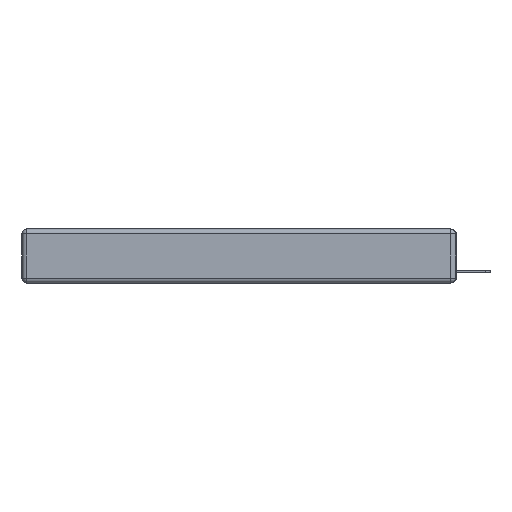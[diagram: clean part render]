
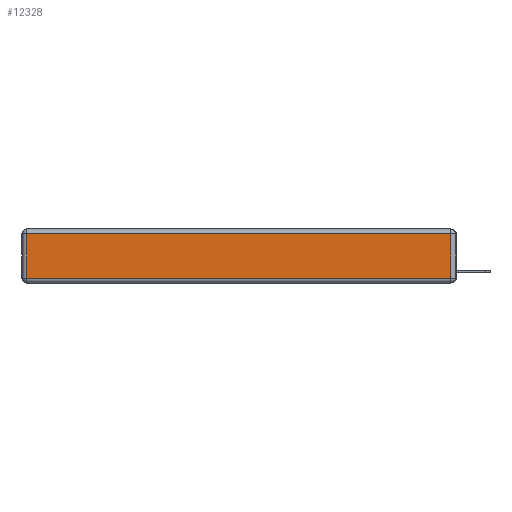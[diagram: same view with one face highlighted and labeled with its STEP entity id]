
A CAD part, left-side view. The second image highlights one B-rep face of the part: STEP entity #12328.
In plain terms, the highlighted planar face has unit normal (-1, 0, 0).
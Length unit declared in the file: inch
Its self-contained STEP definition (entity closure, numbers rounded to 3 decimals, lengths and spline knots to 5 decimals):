
#53 = CARTESIAN_POINT ( 'NONE',  ( 0., 2.72, -0.343 ) ) ;
#652 = LINE ( 'NONE', #5938, #7479 ) ;
#2507 = DIRECTION ( 'NONE',  ( 0., 0., 1. ) ) ;
#4062 = ORIENTED_EDGE ( 'NONE', *, *, #15319, .T. ) ;
#4924 = VECTOR ( 'NONE', #12206, 39.37008 ) ;
#4990 = VERTEX_POINT ( 'NONE', #15341 ) ;
#5711 = EDGE_LOOP ( 'NONE', ( #21194, #4062, #20924, #20977 ) ) ;
#5770 = LINE ( 'NONE', #12170, #21410 ) ;
#5938 = CARTESIAN_POINT ( 'NONE',  ( 0., 0.03, -0.343 ) ) ;
#6281 = VERTEX_POINT ( 'NONE', #16729 ) ;
#6912 = EDGE_CURVE ( 'NONE', #4990, #13314, #8471, .T. ) ;
#7470 = CARTESIAN_POINT ( 'NONE',  ( 0., 0.03, -0.03 ) ) ;
#7479 = VECTOR ( 'NONE', #2507, 39.37008 ) ;
#7860 = DIRECTION ( 'NONE',  ( -1., 0., 0. ) ) ;
#8471 = LINE ( 'NONE', #17300, #4924 ) ;
#8513 = DIRECTION ( 'NONE',  ( 0., 1., 0. ) ) ;
#8737 = CARTESIAN_POINT ( 'NONE',  ( 0., 0.03, -0.313 ) ) ;
#9695 = VERTEX_POINT ( 'NONE', #7470 ) ;
#12170 = CARTESIAN_POINT ( 'NONE',  ( 0., 2.75, -0.03 ) ) ;
#12206 = DIRECTION ( 'NONE',  ( 0., -1., 0. ) ) ;
#12328 = ADVANCED_FACE ( 'NONE', ( #20492 ), #12978, .T. ) ;
#12978 = PLANE ( 'NONE',  #16271 ) ;
#13141 = DIRECTION ( 'NONE',  ( 0., 0., 1. ) ) ;
#13314 = VERTEX_POINT ( 'NONE', #8737 ) ;
#15319 = EDGE_CURVE ( 'NONE', #13314, #9695, #652, .T. ) ;
#15341 = CARTESIAN_POINT ( 'NONE',  ( 0., 2.72, -0.313 ) ) ;
#15437 = LINE ( 'NONE', #53, #18173 ) ;
#15855 = EDGE_CURVE ( 'NONE', #6281, #4990, #15437, .T. ) ;
#16271 = AXIS2_PLACEMENT_3D ( 'NONE', #18284, #7860, #13141 ) ;
#16402 = EDGE_CURVE ( 'NONE', #9695, #6281, #5770, .T. ) ;
#16729 = CARTESIAN_POINT ( 'NONE',  ( 0., 2.72, -0.03 ) ) ;
#17300 = CARTESIAN_POINT ( 'NONE',  ( 0., 0., -0.313 ) ) ;
#18173 = VECTOR ( 'NONE', #19508, 39.37008 ) ;
#18284 = CARTESIAN_POINT ( 'NONE',  ( 0., 0., -0.343 ) ) ;
#19508 = DIRECTION ( 'NONE',  ( 0., 0., -1. ) ) ;
#20492 = FACE_OUTER_BOUND ( 'NONE', #5711, .T. ) ;
#20924 = ORIENTED_EDGE ( 'NONE', *, *, #16402, .T. ) ;
#20977 = ORIENTED_EDGE ( 'NONE', *, *, #15855, .T. ) ;
#21194 = ORIENTED_EDGE ( 'NONE', *, *, #6912, .T. ) ;
#21410 = VECTOR ( 'NONE', #8513, 39.37008 ) ;
